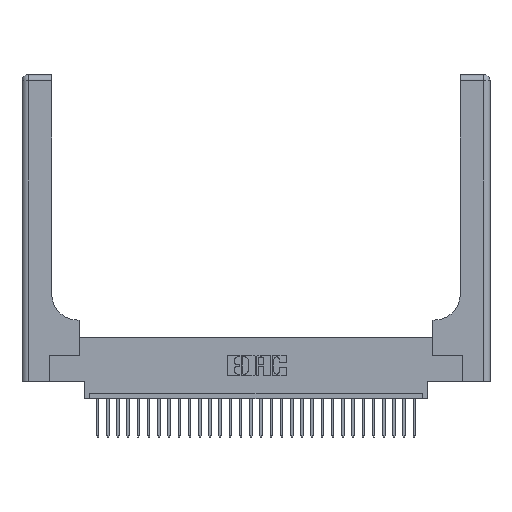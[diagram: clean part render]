
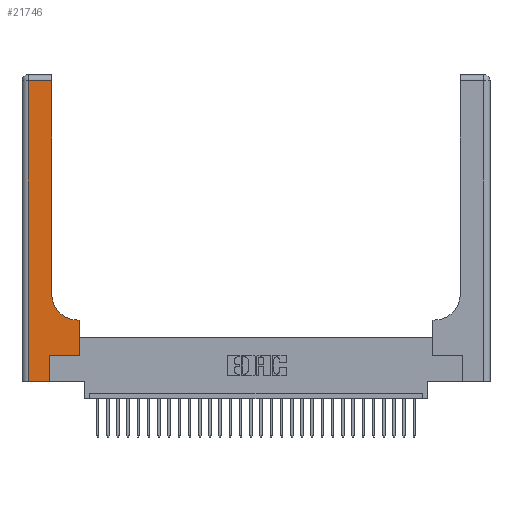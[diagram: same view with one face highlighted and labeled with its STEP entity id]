
A CAD part, top view. The second image highlights one B-rep face of the part: STEP entity #21746.
In plain terms, the highlighted planar face has unit normal (0, 0, 1).
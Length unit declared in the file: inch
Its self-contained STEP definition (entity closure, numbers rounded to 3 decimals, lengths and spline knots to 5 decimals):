
#870 = LINE ( 'NONE', #18859, #25102 ) ;
#1546 = VERTEX_POINT ( 'NONE', #12214 ) ;
#1771 = VECTOR ( 'NONE', #11315, 39.37008 ) ;
#2306 = LINE ( 'NONE', #18516, #21669 ) ;
#3256 = VECTOR ( 'NONE', #5677, 39.37008 ) ;
#3396 = LINE ( 'NONE', #4364, #10056 ) ;
#3907 = EDGE_CURVE ( 'NONE', #1546, #30178, #3396, .T. ) ;
#4364 = CARTESIAN_POINT ( 'NONE',  ( 0., 2.94, 0.37 ) ) ;
#4384 = EDGE_CURVE ( 'NONE', #24524, #14349, #4871, .T. ) ;
#4669 = CARTESIAN_POINT ( 'NONE',  ( 0.269, 0.25, 0.37 ) ) ;
#4871 = LINE ( 'NONE', #21068, #24969 ) ;
#4943 = DIRECTION ( 'NONE',  ( 0., 1., 0. ) ) ;
#5284 = CARTESIAN_POINT ( 'NONE',  ( 0.5585, 0.25, 0.37 ) ) ;
#5677 = DIRECTION ( 'NONE',  ( 0., -1., 0. ) ) ;
#7101 = CARTESIAN_POINT ( 'NONE',  ( 0.5585, 0.25, 0.37 ) ) ;
#7691 = CARTESIAN_POINT ( 'NONE',  ( 0.06, 2.94, 0.37 ) ) ;
#7696 = VECTOR ( 'NONE', #16527, 39.37008 ) ;
#8405 = CARTESIAN_POINT ( 'NONE',  ( 0.5415, 0.85, 0.37 ) ) ;
#9598 = ORIENTED_EDGE ( 'NONE', *, *, #18486, .T. ) ;
#10056 = VECTOR ( 'NONE', #13941, 39.37008 ) ;
#10450 = EDGE_CURVE ( 'NONE', #21261, #30612, #17370, .T. ) ;
#11272 = FACE_OUTER_BOUND ( 'NONE', #12930, .T. ) ;
#11315 = DIRECTION ( 'NONE',  ( 0., 1., 0. ) ) ;
#12214 = CARTESIAN_POINT ( 'NONE',  ( 0.2915, 2.94, 0.37 ) ) ;
#12930 = EDGE_LOOP ( 'NONE', ( #9598, #27936, #16642, #28439, #14924, #27974, #26413, #14167, #22621 ) ) ;
#12948 = LINE ( 'NONE', #18615, #1771 ) ;
#13117 = DIRECTION ( 'NONE',  ( 1., 0., 0. ) ) ;
#13941 = DIRECTION ( 'NONE',  ( -1., 0., 0. ) ) ;
#14005 = PLANE ( 'NONE',  #22968 ) ;
#14167 = ORIENTED_EDGE ( 'NONE', *, *, #4384, .T. ) ;
#14270 = AXIS2_PLACEMENT_3D ( 'NONE', #8405, #20285, #13117 ) ;
#14294 = CARTESIAN_POINT ( 'NONE',  ( 0., 3., 0.37 ) ) ;
#14349 = VERTEX_POINT ( 'NONE', #17827 ) ;
#14694 = DIRECTION ( 'NONE',  ( 0., 0., -1. ) ) ;
#14828 = CARTESIAN_POINT ( 'NONE',  ( 0.5585, 0.6, 0.37 ) ) ;
#14924 = ORIENTED_EDGE ( 'NONE', *, *, #15260, .T. ) ;
#15119 = EDGE_CURVE ( 'NONE', #14349, #23043, #26367, .T. ) ;
#15260 = EDGE_CURVE ( 'NONE', #30342, #21261, #12948, .T. ) ;
#16491 = VERTEX_POINT ( 'NONE', #25207 ) ;
#16527 = DIRECTION ( 'NONE',  ( 1., 0., 0. ) ) ;
#16642 = ORIENTED_EDGE ( 'NONE', *, *, #27689, .T. ) ;
#16664 = DIRECTION ( 'NONE',  ( 1., 0., 0. ) ) ;
#16901 = CARTESIAN_POINT ( 'NONE',  ( 0.2915, 0.85, 0.37 ) ) ;
#17370 = LINE ( 'NONE', #28277, #7696 ) ;
#17527 = CARTESIAN_POINT ( 'NONE',  ( 0.06, 3., 0.37 ) ) ;
#17827 = CARTESIAN_POINT ( 'NONE',  ( 0.5415, 0.6, 0.37 ) ) ;
#18486 = EDGE_CURVE ( 'NONE', #23043, #1546, #2306, .T. ) ;
#18516 = CARTESIAN_POINT ( 'NONE',  ( 0.2915, 3., 0.37 ) ) ;
#18615 = CARTESIAN_POINT ( 'NONE',  ( 0.269, 0., 0.37 ) ) ;
#18859 = CARTESIAN_POINT ( 'NONE',  ( 0., 0., 0.37 ) ) ;
#19328 = LINE ( 'NONE', #7101, #23065 ) ;
#20285 = DIRECTION ( 'NONE',  ( 0., 0., -1. ) ) ;
#20901 = CARTESIAN_POINT ( 'NONE',  ( 0.269, 0., 0.37 ) ) ;
#21068 = CARTESIAN_POINT ( 'NONE',  ( 0.2915, 0.6, 0.37 ) ) ;
#21261 = VERTEX_POINT ( 'NONE', #4669 ) ;
#21669 = VECTOR ( 'NONE', #23316, 39.37008 ) ;
#21746 = ADVANCED_FACE ( 'NONE', ( #11272 ), #14005, .F. ) ;
#22621 = ORIENTED_EDGE ( 'NONE', *, *, #15119, .T. ) ;
#22968 = AXIS2_PLACEMENT_3D ( 'NONE', #14294, #14694, #23854 ) ;
#23043 = VERTEX_POINT ( 'NONE', #16901 ) ;
#23065 = VECTOR ( 'NONE', #4943, 39.37008 ) ;
#23316 = DIRECTION ( 'NONE',  ( 0., 1., 0. ) ) ;
#23854 = DIRECTION ( 'NONE',  ( -1., 0., 0. ) ) ;
#24524 = VERTEX_POINT ( 'NONE', #14828 ) ;
#24825 = EDGE_CURVE ( 'NONE', #30612, #24524, #19328, .T. ) ;
#24969 = VECTOR ( 'NONE', #25541, 39.37008 ) ;
#25102 = VECTOR ( 'NONE', #16664, 39.37008 ) ;
#25207 = CARTESIAN_POINT ( 'NONE',  ( 0.06, 0., 0.37 ) ) ;
#25541 = DIRECTION ( 'NONE',  ( -1., 0., 0. ) ) ;
#26367 = CIRCLE ( 'NONE', #14270, 0.25 ) ;
#26413 = ORIENTED_EDGE ( 'NONE', *, *, #24825, .T. ) ;
#27689 = EDGE_CURVE ( 'NONE', #30178, #16491, #30357, .T. ) ;
#27936 = ORIENTED_EDGE ( 'NONE', *, *, #3907, .T. ) ;
#27974 = ORIENTED_EDGE ( 'NONE', *, *, #10450, .T. ) ;
#28277 = CARTESIAN_POINT ( 'NONE',  ( 0.269, 0.25, 0.37 ) ) ;
#28439 = ORIENTED_EDGE ( 'NONE', *, *, #29797, .T. ) ;
#29797 = EDGE_CURVE ( 'NONE', #16491, #30342, #870, .T. ) ;
#30178 = VERTEX_POINT ( 'NONE', #7691 ) ;
#30342 = VERTEX_POINT ( 'NONE', #20901 ) ;
#30357 = LINE ( 'NONE', #17527, #3256 ) ;
#30612 = VERTEX_POINT ( 'NONE', #5284 ) ;
